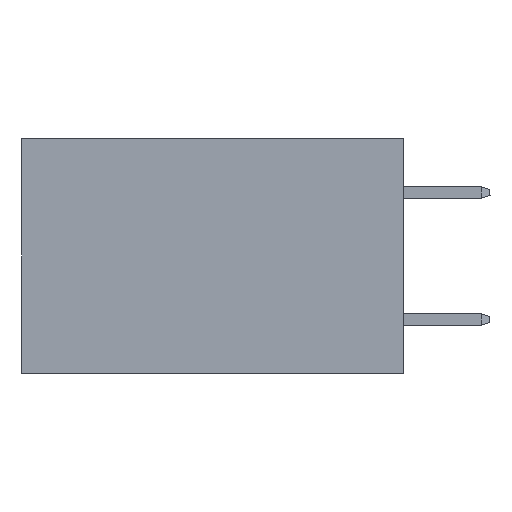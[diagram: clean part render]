
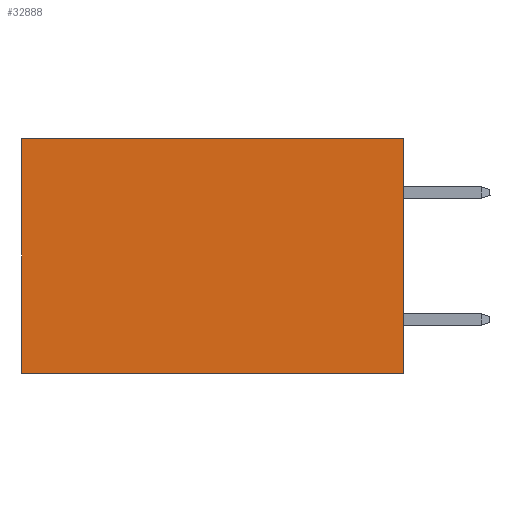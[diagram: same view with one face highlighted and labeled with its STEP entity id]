
A CAD part, left-side view. The second image highlights one B-rep face of the part: STEP entity #32888.
In plain terms, the highlighted planar face has unit normal (-1, 0, 0).
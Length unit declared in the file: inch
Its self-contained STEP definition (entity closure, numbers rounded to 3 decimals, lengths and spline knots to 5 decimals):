
#2212 = CARTESIAN_POINT ( 'NONE',  ( 0.2875, 0., 0. ) ) ;
#2325 = CARTESIAN_POINT ( 'NONE',  ( 0.2875, 0., 0. ) ) ;
#3055 = EDGE_CURVE ( 'NONE', #39021, #11701, #29452, .T. ) ;
#4005 = CARTESIAN_POINT ( 'NONE',  ( 0.2875, 0.6, -0.37 ) ) ;
#4211 = EDGE_CURVE ( 'NONE', #11701, #23296, #25282, .T. ) ;
#7368 = AXIS2_PLACEMENT_3D ( 'NONE', #23994, #36122, #33131 ) ;
#9493 = ORIENTED_EDGE ( 'NONE', *, *, #26122, .F. ) ;
#9775 = LINE ( 'NONE', #29864, #15312 ) ;
#11701 = VERTEX_POINT ( 'NONE', #15142 ) ;
#11877 = PLANE ( 'NONE',  #7368 ) ;
#12498 = LINE ( 'NONE', #21245, #25099 ) ;
#13339 = EDGE_LOOP ( 'NONE', ( #17101, #13987, #9493, #16490 ) ) ;
#13987 = ORIENTED_EDGE ( 'NONE', *, *, #31103, .F. ) ;
#15142 = CARTESIAN_POINT ( 'NONE',  ( 0.2875, 0.6, 0. ) ) ;
#15312 = VECTOR ( 'NONE', #21138, 39.37008 ) ;
#16490 = ORIENTED_EDGE ( 'NONE', *, *, #3055, .T. ) ;
#17101 = ORIENTED_EDGE ( 'NONE', *, *, #4211, .T. ) ;
#18454 = DIRECTION ( 'NONE',  ( 0., 1., 0. ) ) ;
#21138 = DIRECTION ( 'NONE',  ( 0., 0., -1. ) ) ;
#21245 = CARTESIAN_POINT ( 'NONE',  ( 0.2875, 0., -0.37 ) ) ;
#23296 = VERTEX_POINT ( 'NONE', #4005 ) ;
#23994 = CARTESIAN_POINT ( 'NONE',  ( 0.2875, 0., 0. ) ) ;
#25099 = VECTOR ( 'NONE', #18454, 39.37008 ) ;
#25282 = LINE ( 'NONE', #31838, #25782 ) ;
#25782 = VECTOR ( 'NONE', #26075, 39.37008 ) ;
#26075 = DIRECTION ( 'NONE',  ( 0., 0., -1. ) ) ;
#26122 = EDGE_CURVE ( 'NONE', #39021, #31157, #9775, .T. ) ;
#29452 = LINE ( 'NONE', #2212, #30100 ) ;
#29864 = CARTESIAN_POINT ( 'NONE',  ( 0.2875, 0., 0. ) ) ;
#30100 = VECTOR ( 'NONE', #35641, 39.37008 ) ;
#31103 = EDGE_CURVE ( 'NONE', #31157, #23296, #12498, .T. ) ;
#31157 = VERTEX_POINT ( 'NONE', #36175 ) ;
#31838 = CARTESIAN_POINT ( 'NONE',  ( 0.2875, 0.6, 0. ) ) ;
#32888 = ADVANCED_FACE ( 'NONE', ( #39098 ), #11877, .F. ) ;
#33131 = DIRECTION ( 'NONE',  ( 0., 0., -1. ) ) ;
#35641 = DIRECTION ( 'NONE',  ( 0., 1., 0. ) ) ;
#36122 = DIRECTION ( 'NONE',  ( 1., 0., 0. ) ) ;
#36175 = CARTESIAN_POINT ( 'NONE',  ( 0.2875, 0., -0.37 ) ) ;
#39021 = VERTEX_POINT ( 'NONE', #2325 ) ;
#39098 = FACE_OUTER_BOUND ( 'NONE', #13339, .T. ) ;
